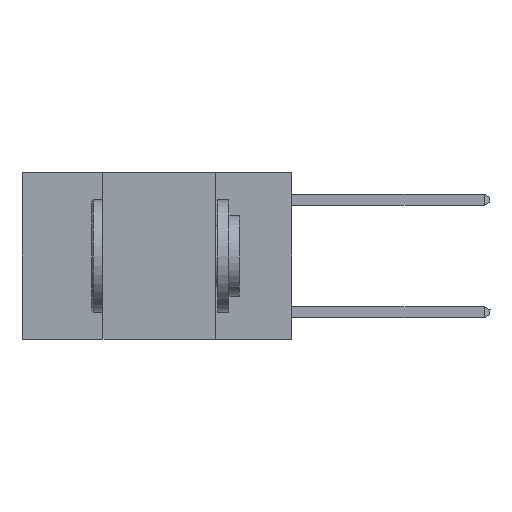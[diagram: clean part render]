
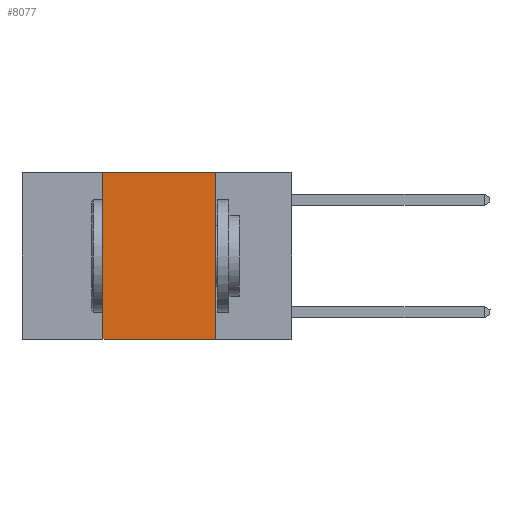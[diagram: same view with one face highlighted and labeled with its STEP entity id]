
A CAD part, left-side view. The second image highlights one B-rep face of the part: STEP entity #8077.
In plain terms, the highlighted planar face has unit normal (-1, 0, 0).
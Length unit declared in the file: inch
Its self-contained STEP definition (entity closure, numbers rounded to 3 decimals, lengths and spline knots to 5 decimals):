
#213 = VECTOR ( 'NONE', #11837, 39.37008 ) ;
#390 = EDGE_CURVE ( 'NONE', #10840, #18157, #13354, .T. ) ;
#1632 = ORIENTED_EDGE ( 'NONE', *, *, #24593, .F. ) ;
#2262 = AXIS2_PLACEMENT_3D ( 'NONE', #9852, #16020, #3246 ) ;
#3246 = DIRECTION ( 'NONE',  ( 0., 0., -1. ) ) ;
#4010 = CARTESIAN_POINT ( 'NONE',  ( 0., 0.17, 0. ) ) ;
#7523 = VECTOR ( 'NONE', #26093, 39.37008 ) ;
#7831 = VECTOR ( 'NONE', #17591, 39.37008 ) ;
#8040 = CARTESIAN_POINT ( 'NONE',  ( 0., 0.17, 0. ) ) ;
#8043 = CARTESIAN_POINT ( 'NONE',  ( 0., 0.42, -0.37 ) ) ;
#8077 = ADVANCED_FACE ( 'NONE', ( #16199 ), #25849, .F. ) ;
#8163 = VERTEX_POINT ( 'NONE', #8040 ) ;
#9349 = EDGE_LOOP ( 'NONE', ( #1632, #13711, #13410, #13972 ) ) ;
#9790 = CARTESIAN_POINT ( 'NONE',  ( 0., 0.42, 0. ) ) ;
#9852 = CARTESIAN_POINT ( 'NONE',  ( 0., 0.6, 0. ) ) ;
#10840 = VERTEX_POINT ( 'NONE', #8043 ) ;
#11837 = DIRECTION ( 'NONE',  ( 0., 0., 1. ) ) ;
#13072 = LINE ( 'NONE', #22243, #7523 ) ;
#13354 = LINE ( 'NONE', #17897, #7831 ) ;
#13410 = ORIENTED_EDGE ( 'NONE', *, *, #20630, .F. ) ;
#13711 = ORIENTED_EDGE ( 'NONE', *, *, #18971, .F. ) ;
#13972 = ORIENTED_EDGE ( 'NONE', *, *, #390, .T. ) ;
#16020 = DIRECTION ( 'NONE',  ( 1., 0., 0. ) ) ;
#16048 = CARTESIAN_POINT ( 'NONE',  ( 0., 0.17, -0.37 ) ) ;
#16199 = FACE_OUTER_BOUND ( 'NONE', #9349, .T. ) ;
#16597 = VECTOR ( 'NONE', #26465, 39.37008 ) ;
#17591 = DIRECTION ( 'NONE',  ( 0., -1., 0. ) ) ;
#17897 = CARTESIAN_POINT ( 'NONE',  ( 0., 0.6, -0.37 ) ) ;
#18157 = VERTEX_POINT ( 'NONE', #16048 ) ;
#18971 = EDGE_CURVE ( 'NONE', #26248, #8163, #13072, .T. ) ;
#20630 = EDGE_CURVE ( 'NONE', #10840, #26248, #23072, .T. ) ;
#21310 = LINE ( 'NONE', #4010, #16597 ) ;
#22243 = CARTESIAN_POINT ( 'NONE',  ( 0., 0.6, 0. ) ) ;
#22373 = CARTESIAN_POINT ( 'NONE',  ( 0., 0.42, 0. ) ) ;
#23072 = LINE ( 'NONE', #9790, #213 ) ;
#24593 = EDGE_CURVE ( 'NONE', #8163, #18157, #21310, .T. ) ;
#25849 = PLANE ( 'NONE',  #2262 ) ;
#26093 = DIRECTION ( 'NONE',  ( 0., -1., 0. ) ) ;
#26248 = VERTEX_POINT ( 'NONE', #22373 ) ;
#26465 = DIRECTION ( 'NONE',  ( 0., 0., -1. ) ) ;
